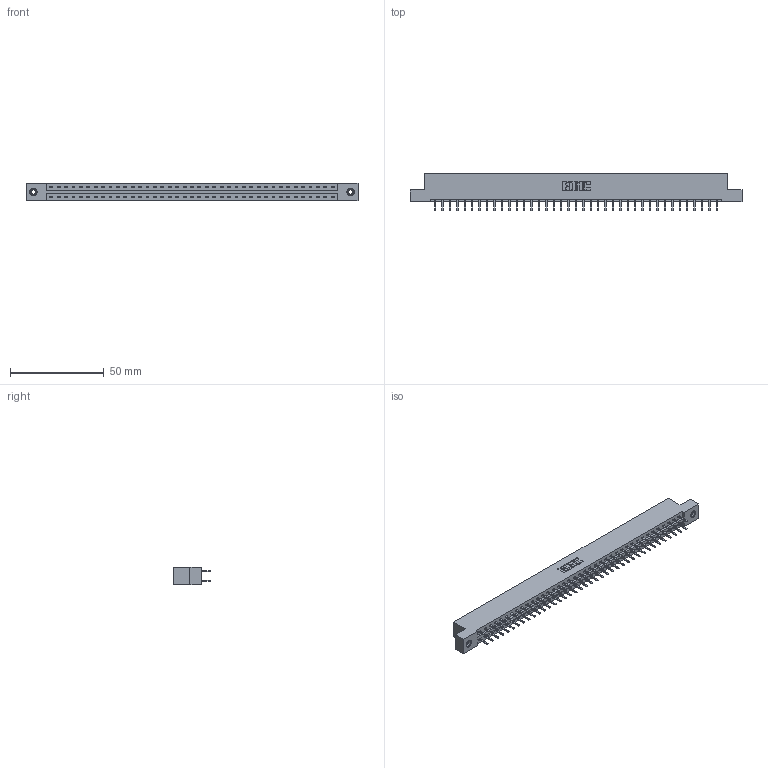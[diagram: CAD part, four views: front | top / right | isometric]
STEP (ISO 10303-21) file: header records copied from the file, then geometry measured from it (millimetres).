
FILE_DESCRIPTION (( 'STEP AP203' ), '1' );
FILE_NAME ('337-078-520-208.STEP', '2019-10-10T11:10:00', ( '' ), ( '' ), 'SwSTEP 2.0', 'SolidWorks 2016', '' );
FILE_SCHEMA (( 'CONFIG_CONTROL_DESIGN' ));
Length unit declared in the file: inch
Products named in the file (4): 337 Part_Flush Mounting Lugs - 0.156 Dia-TI; 345-250-001_345-250-003-102; 337-078-520-208; 345-292-001_345-293-120
Assembly tree (81 placements, depth 2):
  337-078-520-208
    337 Part_Flush Mounting Lugs - 0.156 Dia-TI
    345-292-001_345-293-120  x78
    345-250-001_345-250-003-102  x2
Bounding box: 177.55 x 20.02 x 9.4 mm (x, y, z)
Volume: 18630.5 mm3; surface area: 20958.8 mm2
Topology: 81 solids, 81 shells, 4698 faces, 13629 edges, 8870 vertices
Faces by surface type: plane 3222, cylinder 1460, cone 12, torus 4
Entity records: 31926 total; most frequent: CARTESIAN_POINT 5373, ORIENTED_EDGE 5290, DIRECTION 4595, EDGE_CURVE 2645, LINE 2493, VECTOR 2493, VERTEX_POINT 1756, AXIS2_PLACEMENT_3D 1051
